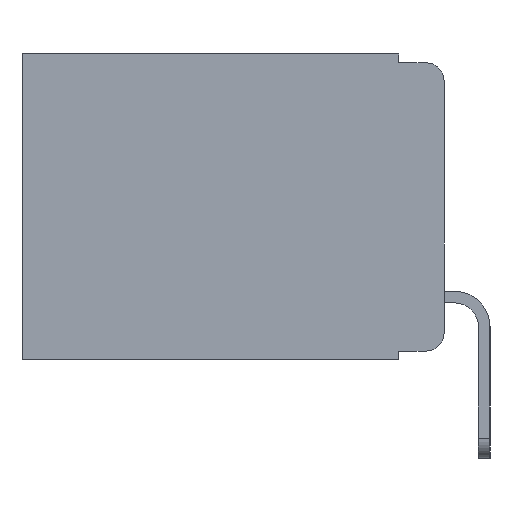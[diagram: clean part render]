
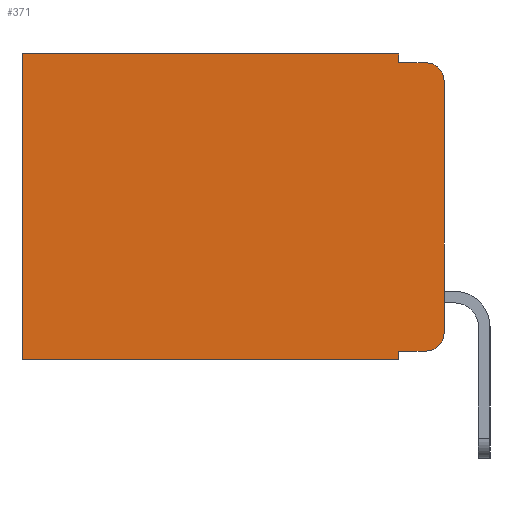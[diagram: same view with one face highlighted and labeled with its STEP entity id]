
A CAD part, left-side view. The second image highlights one B-rep face of the part: STEP entity #371.
In plain terms, the highlighted planar face has unit normal (-1, 0, 0).
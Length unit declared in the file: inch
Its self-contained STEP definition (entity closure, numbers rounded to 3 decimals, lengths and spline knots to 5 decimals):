
#8 = DIRECTION ( 'NONE',  ( 0., -1., 0. ) ) ;
#371 = ADVANCED_FACE ( 'NONE', ( #3328 ), #4197, .F. ) ;
#927 = ORIENTED_EDGE ( 'NONE', *, *, #17657, .F. ) ;
#1342 = ORIENTED_EDGE ( 'NONE', *, *, #17431, .F. ) ;
#1550 = VECTOR ( 'NONE', #10639, 39.37008 ) ;
#1984 = EDGE_LOOP ( 'NONE', ( #14348, #13245, #3764, #2561, #4256, #7275, #1342, #927, #8331, #12414 ) ) ;
#2381 = EDGE_CURVE ( 'NONE', #13907, #2481, #20358, .T. ) ;
#2481 = VERTEX_POINT ( 'NONE', #7074 ) ;
#2561 = ORIENTED_EDGE ( 'NONE', *, *, #9815, .F. ) ;
#2648 = AXIS2_PLACEMENT_3D ( 'NONE', #17197, #11020, #8214 ) ;
#2765 = VECTOR ( 'NONE', #18058, 39.37008 ) ;
#2923 = CARTESIAN_POINT ( 'NONE',  ( 0.298, 0.473, 0. ) ) ;
#3328 = FACE_OUTER_BOUND ( 'NONE', #1984, .T. ) ;
#3764 = ORIENTED_EDGE ( 'NONE', *, *, #18596, .F. ) ;
#4125 = CARTESIAN_POINT ( 'NONE',  ( 0.298, 0.02, -0.333 ) ) ;
#4197 = PLANE ( 'NONE',  #2648 ) ;
#4242 = VECTOR ( 'NONE', #18153, 39.37008 ) ;
#4256 = ORIENTED_EDGE ( 'NONE', *, *, #16799, .T. ) ;
#5724 = VECTOR ( 'NONE', #11030, 39.37008 ) ;
#5795 = CARTESIAN_POINT ( 'NONE',  ( 0.298, 0.051, 0. ) ) ;
#7074 = CARTESIAN_POINT ( 'NONE',  ( 0.298, 0.02, -0.01 ) ) ;
#7275 = ORIENTED_EDGE ( 'NONE', *, *, #18713, .T. ) ;
#7312 = CARTESIAN_POINT ( 'NONE',  ( 0.298, 0., 0. ) ) ;
#7445 = CARTESIAN_POINT ( 'NONE',  ( 0.298, 0.051, 0. ) ) ;
#8054 = VECTOR ( 'NONE', #20071, 39.37008 ) ;
#8214 = DIRECTION ( 'NONE',  ( 0., 0., -1. ) ) ;
#8282 = DIRECTION ( 'NONE',  ( 0., 0., -1. ) ) ;
#8321 = LINE ( 'NONE', #2923, #2765 ) ;
#8331 = ORIENTED_EDGE ( 'NONE', *, *, #9151, .T. ) ;
#9095 = VERTEX_POINT ( 'NONE', #9326 ) ;
#9151 = EDGE_CURVE ( 'NONE', #9095, #17700, #18090, .T. ) ;
#9291 = CARTESIAN_POINT ( 'NONE',  ( 0.298, 0.02, -0.313 ) ) ;
#9326 = CARTESIAN_POINT ( 'NONE',  ( 0.298, 0.051, -0.333 ) ) ;
#9815 = EDGE_CURVE ( 'NONE', #21902, #15876, #15902, .T. ) ;
#9840 = LINE ( 'NONE', #19276, #17797 ) ;
#10518 = VECTOR ( 'NONE', #11125, 39.37008 ) ;
#10639 = DIRECTION ( 'NONE',  ( 0., 0., -1. ) ) ;
#10697 = CARTESIAN_POINT ( 'NONE',  ( 0.298, 0.473, 0. ) ) ;
#10703 = AXIS2_PLACEMENT_3D ( 'NONE', #9291, #20333, #10904 ) ;
#10904 = DIRECTION ( 'NONE',  ( 0., 0., -1. ) ) ;
#10924 = CARTESIAN_POINT ( 'NONE',  ( 0.298, 0.473, -0.343 ) ) ;
#10948 = DIRECTION ( 'NONE',  ( -1., 0., 0. ) ) ;
#10967 = CARTESIAN_POINT ( 'NONE',  ( 0.298, 0.02, -0.03 ) ) ;
#11020 = DIRECTION ( 'NONE',  ( 1., 0., 0. ) ) ;
#11030 = DIRECTION ( 'NONE',  ( 0., 0., -1. ) ) ;
#11125 = DIRECTION ( 'NONE',  ( 0., 0., -1. ) ) ;
#11333 = LINE ( 'NONE', #5795, #5724 ) ;
#11409 = DIRECTION ( 'NONE',  ( 0., -1., 0. ) ) ;
#11866 = EDGE_CURVE ( 'NONE', #13907, #14398, #14329, .T. ) ;
#12414 = ORIENTED_EDGE ( 'NONE', *, *, #21149, .T. ) ;
#12590 = CARTESIAN_POINT ( 'NONE',  ( 0.298, 0.051, -0.333 ) ) ;
#13245 = ORIENTED_EDGE ( 'NONE', *, *, #2381, .T. ) ;
#13411 = LINE ( 'NONE', #13542, #4242 ) ;
#13542 = CARTESIAN_POINT ( 'NONE',  ( 0.298, 0., -0.343 ) ) ;
#13729 = VERTEX_POINT ( 'NONE', #19588 ) ;
#13907 = VERTEX_POINT ( 'NONE', #21651 ) ;
#13950 = VECTOR ( 'NONE', #8, 39.37008 ) ;
#14329 = LINE ( 'NONE', #17415, #10518 ) ;
#14348 = ORIENTED_EDGE ( 'NONE', *, *, #11866, .F. ) ;
#14398 = VERTEX_POINT ( 'NONE', #16255 ) ;
#15876 = VERTEX_POINT ( 'NONE', #21092 ) ;
#15902 = LINE ( 'NONE', #21609, #1550 ) ;
#16001 = AXIS2_PLACEMENT_3D ( 'NONE', #10967, #10948, #8282 ) ;
#16255 = CARTESIAN_POINT ( 'NONE',  ( 0.298, 0., -0.313 ) ) ;
#16799 = EDGE_CURVE ( 'NONE', #21902, #16839, #20681, .T. ) ;
#16839 = VERTEX_POINT ( 'NONE', #10697 ) ;
#17197 = CARTESIAN_POINT ( 'NONE',  ( 0.298, 0., 0. ) ) ;
#17415 = CARTESIAN_POINT ( 'NONE',  ( 0.298, 0., 0. ) ) ;
#17431 = EDGE_CURVE ( 'NONE', #13729, #19148, #13411, .T. ) ;
#17657 = EDGE_CURVE ( 'NONE', #9095, #13729, #11333, .T. ) ;
#17700 = VERTEX_POINT ( 'NONE', #4125 ) ;
#17797 = VECTOR ( 'NONE', #11409, 39.37008 ) ;
#18058 = DIRECTION ( 'NONE',  ( 0., 0., -1. ) ) ;
#18090 = LINE ( 'NONE', #12590, #13950 ) ;
#18153 = DIRECTION ( 'NONE',  ( 0., 1., 0. ) ) ;
#18212 = CIRCLE ( 'NONE', #10703, 0.02 ) ;
#18596 = EDGE_CURVE ( 'NONE', #15876, #2481, #9840, .T. ) ;
#18713 = EDGE_CURVE ( 'NONE', #16839, #19148, #8321, .T. ) ;
#19148 = VERTEX_POINT ( 'NONE', #10924 ) ;
#19276 = CARTESIAN_POINT ( 'NONE',  ( 0.298, 0.051, -0.01 ) ) ;
#19588 = CARTESIAN_POINT ( 'NONE',  ( 0.298, 0.051, -0.343 ) ) ;
#20071 = DIRECTION ( 'NONE',  ( 0., 1., 0. ) ) ;
#20333 = DIRECTION ( 'NONE',  ( -1., 0., 0. ) ) ;
#20358 = CIRCLE ( 'NONE', #16001, 0.02 ) ;
#20681 = LINE ( 'NONE', #7312, #8054 ) ;
#21092 = CARTESIAN_POINT ( 'NONE',  ( 0.298, 0.051, -0.01 ) ) ;
#21149 = EDGE_CURVE ( 'NONE', #17700, #14398, #18212, .T. ) ;
#21609 = CARTESIAN_POINT ( 'NONE',  ( 0.298, 0.051, 0. ) ) ;
#21651 = CARTESIAN_POINT ( 'NONE',  ( 0.298, 0., -0.03 ) ) ;
#21902 = VERTEX_POINT ( 'NONE', #7445 ) ;
